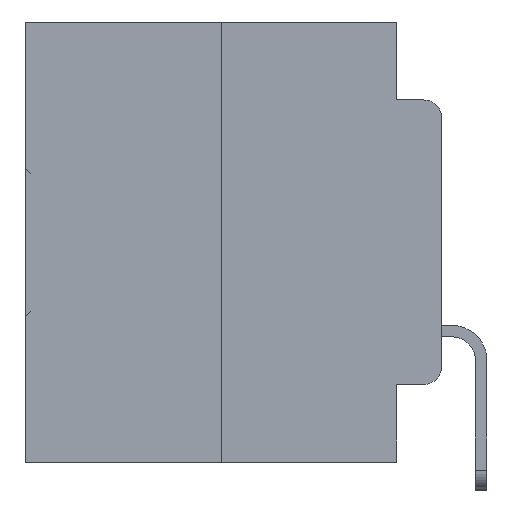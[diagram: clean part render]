
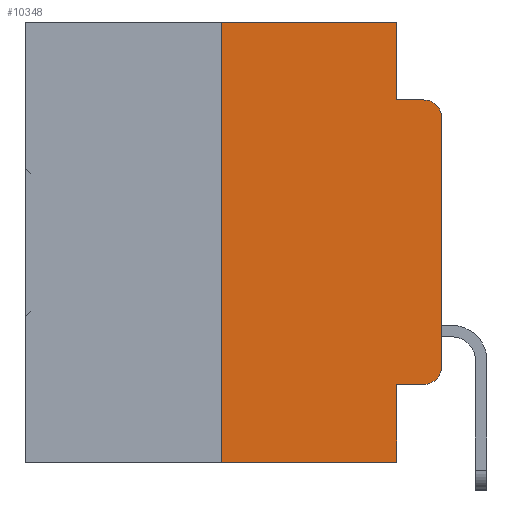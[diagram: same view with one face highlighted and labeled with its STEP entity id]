
A CAD part, left-side view. The second image highlights one B-rep face of the part: STEP entity #10348.
In plain terms, the highlighted planar face has unit normal (-1, 0, 0).
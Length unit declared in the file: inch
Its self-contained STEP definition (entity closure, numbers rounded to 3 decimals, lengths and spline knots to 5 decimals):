
#122 = VERTEX_POINT ( 'NONE', #10922 ) ;
#877 = EDGE_CURVE ( 'NONE', #1604, #1546, #13800, .T. ) ;
#1016 = EDGE_CURVE ( 'NONE', #24039, #19298, #16532, .T. ) ;
#1454 = VECTOR ( 'NONE', #12145, 39.37008 ) ;
#1546 = VERTEX_POINT ( 'NONE', #4413 ) ;
#1604 = VERTEX_POINT ( 'NONE', #16322 ) ;
#1862 = EDGE_CURVE ( 'NONE', #20099, #1546, #10625, .T. ) ;
#2006 = AXIS2_PLACEMENT_3D ( 'NONE', #12189, #29457, #14723 ) ;
#2432 = VECTOR ( 'NONE', #16348, 39.37008 ) ;
#3237 = CARTESIAN_POINT ( 'NONE',  ( 0., 0.02, -0.3915 ) ) ;
#3601 = CARTESIAN_POINT ( 'NONE',  ( 0., 0.051, -0.4115 ) ) ;
#3897 = VECTOR ( 'NONE', #17072, 39.37008 ) ;
#4413 = CARTESIAN_POINT ( 'NONE',  ( 0., 0.02, -0.0885 ) ) ;
#4560 = ORIENTED_EDGE ( 'NONE', *, *, #20424, .T. ) ;
#5077 = VECTOR ( 'NONE', #22738, 39.37008 ) ;
#5592 = FACE_OUTER_BOUND ( 'NONE', #31379, .T. ) ;
#5868 = DIRECTION ( 'NONE',  ( 0., 0., -1. ) ) ;
#5968 = VECTOR ( 'NONE', #31534, 39.37008 ) ;
#5995 = EDGE_CURVE ( 'NONE', #15530, #1604, #23268, .T. ) ;
#6033 = EDGE_CURVE ( 'NONE', #24039, #9520, #22474, .T. ) ;
#7173 = PLANE ( 'NONE',  #2006 ) ;
#7187 = ORIENTED_EDGE ( 'NONE', *, *, #7875, .F. ) ;
#7490 = LINE ( 'NONE', #9800, #1454 ) ;
#7848 = CARTESIAN_POINT ( 'NONE',  ( 0., 0.25, 0. ) ) ;
#7875 = EDGE_CURVE ( 'NONE', #30103, #15530, #12619, .T. ) ;
#8488 = CARTESIAN_POINT ( 'NONE',  ( 0., 0.051, 0. ) ) ;
#8510 = VECTOR ( 'NONE', #28728, 39.37008 ) ;
#8935 = AXIS2_PLACEMENT_3D ( 'NONE', #25641, #25572, #23238 ) ;
#9048 = CARTESIAN_POINT ( 'NONE',  ( 0., 0.02, -0.4115 ) ) ;
#9399 = CARTESIAN_POINT ( 'NONE',  ( 0., 0.473, 0. ) ) ;
#9520 = VERTEX_POINT ( 'NONE', #9048 ) ;
#9634 = EDGE_CURVE ( 'NONE', #23796, #20099, #20897, .T. ) ;
#9800 = CARTESIAN_POINT ( 'NONE',  ( 0., 0.473, -0.5 ) ) ;
#10348 = ADVANCED_FACE ( 'NONE', ( #5592 ), #7173, .F. ) ;
#10625 = CIRCLE ( 'NONE', #8935, 0.02 ) ;
#10922 = CARTESIAN_POINT ( 'NONE',  ( 0., 0.25, -0.5 ) ) ;
#12145 = DIRECTION ( 'NONE',  ( 0., -1., 0. ) ) ;
#12189 = CARTESIAN_POINT ( 'NONE',  ( 0., 0.473, 0. ) ) ;
#12444 = ORIENTED_EDGE ( 'NONE', *, *, #5995, .F. ) ;
#12580 = CARTESIAN_POINT ( 'NONE',  ( 0., 0., -0.3915 ) ) ;
#12619 = LINE ( 'NONE', #9399, #5968 ) ;
#12654 = ORIENTED_EDGE ( 'NONE', *, *, #26802, .F. ) ;
#13505 = VECTOR ( 'NONE', #26690, 39.37008 ) ;
#13800 = LINE ( 'NONE', #27603, #20410 ) ;
#14102 = AXIS2_PLACEMENT_3D ( 'NONE', #3237, #20834, #5868 ) ;
#14353 = ORIENTED_EDGE ( 'NONE', *, *, #6033, .T. ) ;
#14723 = DIRECTION ( 'NONE',  ( 0., 0., -1. ) ) ;
#15108 = DIRECTION ( 'NONE',  ( 0., -1., 0. ) ) ;
#15530 = VERTEX_POINT ( 'NONE', #8488 ) ;
#15881 = ORIENTED_EDGE ( 'NONE', *, *, #1862, .T. ) ;
#16060 = EDGE_CURVE ( 'NONE', #9520, #23796, #18442, .T. ) ;
#16322 = CARTESIAN_POINT ( 'NONE',  ( 0., 0.051, -0.0885 ) ) ;
#16348 = DIRECTION ( 'NONE',  ( 0., 0., -1. ) ) ;
#16532 = LINE ( 'NONE', #17102, #3897 ) ;
#16985 = ORIENTED_EDGE ( 'NONE', *, *, #877, .F. ) ;
#17072 = DIRECTION ( 'NONE',  ( 0., 0., -1. ) ) ;
#17102 = CARTESIAN_POINT ( 'NONE',  ( 0., 0.051, 0. ) ) ;
#18442 = CIRCLE ( 'NONE', #14102, 0.02 ) ;
#18964 = ORIENTED_EDGE ( 'NONE', *, *, #1016, .F. ) ;
#19298 = VERTEX_POINT ( 'NONE', #32199 ) ;
#19335 = CARTESIAN_POINT ( 'NONE',  ( 0., 0., 0. ) ) ;
#20099 = VERTEX_POINT ( 'NONE', #28408 ) ;
#20410 = VECTOR ( 'NONE', #15108, 39.37008 ) ;
#20424 = EDGE_CURVE ( 'NONE', #122, #19298, #7490, .T. ) ;
#20834 = DIRECTION ( 'NONE',  ( -1., 0., 0. ) ) ;
#20897 = LINE ( 'NONE', #19335, #13505 ) ;
#21334 = CARTESIAN_POINT ( 'NONE',  ( 0., 0.051, -0.4115 ) ) ;
#22336 = ORIENTED_EDGE ( 'NONE', *, *, #16060, .T. ) ;
#22474 = LINE ( 'NONE', #21334, #8510 ) ;
#22738 = DIRECTION ( 'NONE',  ( 0., 0., 1. ) ) ;
#23238 = DIRECTION ( 'NONE',  ( 0., 0., -1. ) ) ;
#23268 = LINE ( 'NONE', #26197, #2432 ) ;
#23796 = VERTEX_POINT ( 'NONE', #12580 ) ;
#24039 = VERTEX_POINT ( 'NONE', #3601 ) ;
#25572 = DIRECTION ( 'NONE',  ( -1., 0., 0. ) ) ;
#25641 = CARTESIAN_POINT ( 'NONE',  ( 0., 0.02, -0.1085 ) ) ;
#26197 = CARTESIAN_POINT ( 'NONE',  ( 0., 0.051, 0. ) ) ;
#26690 = DIRECTION ( 'NONE',  ( 0., 0., 1. ) ) ;
#26802 = EDGE_CURVE ( 'NONE', #122, #30103, #30677, .T. ) ;
#27603 = CARTESIAN_POINT ( 'NONE',  ( 0., 0.051, -0.0885 ) ) ;
#27948 = CARTESIAN_POINT ( 'NONE',  ( 0., 0.25, 0. ) ) ;
#28408 = CARTESIAN_POINT ( 'NONE',  ( 0., 0., -0.1085 ) ) ;
#28728 = DIRECTION ( 'NONE',  ( 0., -1., 0. ) ) ;
#29457 = DIRECTION ( 'NONE',  ( 1., 0., 0. ) ) ;
#30103 = VERTEX_POINT ( 'NONE', #27948 ) ;
#30123 = ORIENTED_EDGE ( 'NONE', *, *, #9634, .T. ) ;
#30677 = LINE ( 'NONE', #7848, #5077 ) ;
#31379 = EDGE_LOOP ( 'NONE', ( #30123, #15881, #16985, #12444, #7187, #12654, #4560, #18964, #14353, #22336 ) ) ;
#31534 = DIRECTION ( 'NONE',  ( 0., -1., 0. ) ) ;
#32199 = CARTESIAN_POINT ( 'NONE',  ( 0., 0.051, -0.5 ) ) ;
